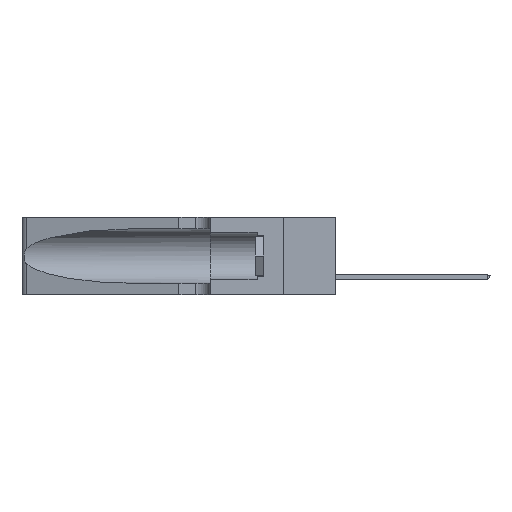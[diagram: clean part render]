
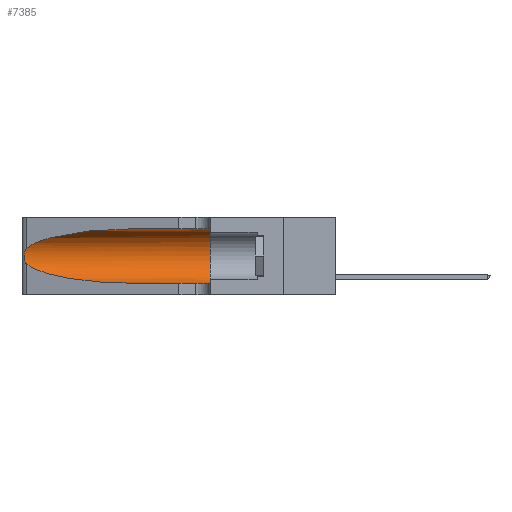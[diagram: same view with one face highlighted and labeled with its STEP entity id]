
A CAD part, left-side view. The second image highlights one B-rep face of the part: STEP entity #7385.
In plain terms, the highlighted cylindrical face has radius 3.308 mm (diameter 6.617 mm), a partial arc.
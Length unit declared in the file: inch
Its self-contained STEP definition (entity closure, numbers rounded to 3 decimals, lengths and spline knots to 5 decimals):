
#1505 = EDGE_CURVE ( 'NONE', #21338, #16410, #26959, .T. ) ;
#1659 = CARTESIAN_POINT ( 'NONE',  ( 0.25555, 1.22994, 0.2215 ) ) ;
#1779 = ORIENTED_EDGE ( 'NONE', *, *, #14193, .F. ) ;
#1918 = DIRECTION ( 'NONE',  ( 0., 0., 1. ) ) ;
#2112 = CARTESIAN_POINT ( 'NONE',  ( 0.1305, 0.35, 0.185 ) ) ;
#3298 = VECTOR ( 'NONE', #12428, 39.37008 ) ;
#4605 = DIRECTION ( 'NONE',  ( 0., -1., 0. ) ) ;
#4845 = VECTOR ( 'NONE', #4605, 39.37008 ) ;
#5491 = ORIENTED_EDGE ( 'NONE', *, *, #15686, .T. ) ;
#5978 = AXIS2_PLACEMENT_3D ( 'NONE', #20679, #14130, #18639 ) ;
#6542 = EDGE_CURVE ( 'NONE', #26342, #21338, #17304, .T. ) ;
#7385 = ADVANCED_FACE ( 'NONE', ( #24668 ), #21579, .F. ) ;
#7404 = CARTESIAN_POINT ( 'NONE',  ( 0.25487, 1.22718, 0.14631 ) ) ;
#8279 = CIRCLE ( 'NONE', #8718, 0.13025 ) ;
#8718 = AXIS2_PLACEMENT_3D ( 'NONE', #2112, #21785, #1918 ) ;
#9043 = CARTESIAN_POINT ( 'NONE',  ( 0.26018, 1.23835, 0.19895 ) ) ;
#9511 = VERTEX_POINT ( 'NONE', #19575 ) ;
#10541 = CARTESIAN_POINT ( 'NONE',  ( 0.25787, 1.23484, 0.2124 ) ) ;
#11440 = CARTESIAN_POINT ( 'NONE',  ( 0.25856, 1.23593, 0.16098 ) ) ;
#11745 = CARTESIAN_POINT ( 'NONE',  ( 0.25487, 1.22718, 0.14631 ) ) ;
#12428 = DIRECTION ( 'NONE',  ( 0., -1., 0. ) ) ;
#12662 = CARTESIAN_POINT ( 'NONE',  ( 0.25487, 1.22718, 0.22369 ) ) ;
#13895 = EDGE_CURVE ( 'NONE', #27005, #9511, #27079, .T. ) ;
#14060 = CARTESIAN_POINT ( 'NONE',  ( 0.1305, 0.35, 0.31525 ) ) ;
#14130 = DIRECTION ( 'NONE',  ( 0., -1., 0. ) ) ;
#14166 = CARTESIAN_POINT ( 'NONE',  ( 0.1305, 0.35, 0.05475 ) ) ;
#14193 = EDGE_CURVE ( 'NONE', #17290, #16410, #8279, .T. ) ;
#15313 = CARTESIAN_POINT ( 'NONE',  ( 0.18966, 0.96281, 0.31525 ) ) ;
#15686 = EDGE_CURVE ( 'NONE', #9511, #26342, #21558, .T. ) ;
#15891 = CARTESIAN_POINT ( 'NONE',  ( 0.25555, 1.22993, 0.14849 ) ) ;
#16410 = VERTEX_POINT ( 'NONE', #14166 ) ;
#17000 = EDGE_CURVE ( 'NONE', #27005, #17290, #21224, .T. ) ;
#17290 = VERTEX_POINT ( 'NONE', #14060 ) ;
#17304 =( BOUNDED_CURVE ( )  B_SPLINE_CURVE ( 3, ( #18963, #27688, #27476, #18769 ),
 .UNSPECIFIED., .F., .F. ) 
 B_SPLINE_CURVE_WITH_KNOTS ( ( 4, 4 ),
 ( 3.44316, 4.71239 ),
 .UNSPECIFIED. ) 
 CURVE ( )  GEOMETRIC_REPRESENTATION_ITEM ( )  RATIONAL_B_SPLINE_CURVE ( ( 1., 0.87, 0.87, 1. ) ) 
 REPRESENTATION_ITEM ( '' )  );
#18005 = CARTESIAN_POINT ( 'NONE',  ( 0.26075, 1.23896, 0.178 ) ) ;
#18448 = EDGE_LOOP ( 'NONE', ( #21596, #5491, #19711, #19684, #1779, #24185 ) ) ;
#18639 = DIRECTION ( 'NONE',  ( 0., 0., -1. ) ) ;
#18769 = CARTESIAN_POINT ( 'NONE',  ( 0.1305, 0.72297, 0.05475 ) ) ;
#18963 = CARTESIAN_POINT ( 'NONE',  ( 0.25487, 1.22718, 0.14631 ) ) ;
#19535 = CARTESIAN_POINT ( 'NONE',  ( 0.2373, 1.15595, 0.28018 ) ) ;
#19575 = CARTESIAN_POINT ( 'NONE',  ( 0.25487, 1.22718, 0.22369 ) ) ;
#19684 = ORIENTED_EDGE ( 'NONE', *, *, #1505, .T. ) ;
#19711 = ORIENTED_EDGE ( 'NONE', *, *, #6542, .T. ) ;
#20114 = CARTESIAN_POINT ( 'NONE',  ( 0.1305, 1.61858, 0.05475 ) ) ;
#20205 = CARTESIAN_POINT ( 'NONE',  ( 0.1305, 0.72297, 0.31525 ) ) ;
#20229 = CARTESIAN_POINT ( 'NONE',  ( 0.26017, 1.23833, 0.17102 ) ) ;
#20679 = CARTESIAN_POINT ( 'NONE',  ( 0.1305, 1.61858, 0.185 ) ) ;
#21147 = CARTESIAN_POINT ( 'NONE',  ( 0.1305, 0.72297, 0.05475 ) ) ;
#21224 = LINE ( 'NONE', #23540, #3298 ) ;
#21338 = VERTEX_POINT ( 'NONE', #21147 ) ;
#21540 = CARTESIAN_POINT ( 'NONE',  ( 0.25639, 1.23184, 0.21858 ) ) ;
#21558 = B_SPLINE_CURVE_WITH_KNOTS ( 'NONE', 3,
 ( #12662, #1659, #21540, #10541, #26028, #9043, #24572, #18005, #20229, #11440, #22531, #26936, #15891, #7404 ),
 .UNSPECIFIED., .F., .F.,
 ( 4, 2, 2, 2, 2, 2, 4 ),
 ( 0., 0.00027, 0.00053, 0.00107, 0.0016, 0.00187, 0.00214 ),
 .UNSPECIFIED. ) ;
#21579 = CYLINDRICAL_SURFACE ( 'NONE', #5978, 0.13025 ) ;
#21596 = ORIENTED_EDGE ( 'NONE', *, *, #13895, .T. ) ;
#21785 = DIRECTION ( 'NONE',  ( 0., 1., 0. ) ) ;
#22531 = CARTESIAN_POINT ( 'NONE',  ( 0.25789, 1.23486, 0.15765 ) ) ;
#23540 = CARTESIAN_POINT ( 'NONE',  ( 0.1305, 1.61858, 0.31525 ) ) ;
#24185 = ORIENTED_EDGE ( 'NONE', *, *, #17000, .F. ) ;
#24572 = CARTESIAN_POINT ( 'NONE',  ( 0.26075, 1.23896, 0.19203 ) ) ;
#24668 = FACE_OUTER_BOUND ( 'NONE', #18448, .T. ) ;
#26028 = CARTESIAN_POINT ( 'NONE',  ( 0.25854, 1.2359, 0.20912 ) ) ;
#26159 = CARTESIAN_POINT ( 'NONE',  ( 0.1305, 0.72297, 0.31525 ) ) ;
#26342 = VERTEX_POINT ( 'NONE', #11745 ) ;
#26808 = CARTESIAN_POINT ( 'NONE',  ( 0.25487, 1.22718, 0.22369 ) ) ;
#26936 = CARTESIAN_POINT ( 'NONE',  ( 0.25639, 1.23186, 0.15144 ) ) ;
#26959 = LINE ( 'NONE', #20114, #4845 ) ;
#27005 = VERTEX_POINT ( 'NONE', #20205 ) ;
#27079 =( BOUNDED_CURVE ( )  B_SPLINE_CURVE ( 3, ( #26159, #15313, #19535, #26808 ),
 .UNSPECIFIED., .F., .T. ) 
 B_SPLINE_CURVE_WITH_KNOTS ( ( 4, 4 ),
 ( 1.5708, 2.84003 ),
 .UNSPECIFIED. ) 
 CURVE ( )  GEOMETRIC_REPRESENTATION_ITEM ( )  RATIONAL_B_SPLINE_CURVE ( ( 1., 0.87, 0.87, 1. ) ) 
 REPRESENTATION_ITEM ( '' )  );
#27476 = CARTESIAN_POINT ( 'NONE',  ( 0.18966, 0.96281, 0.05475 ) ) ;
#27688 = CARTESIAN_POINT ( 'NONE',  ( 0.2373, 1.15595, 0.08982 ) ) ;
